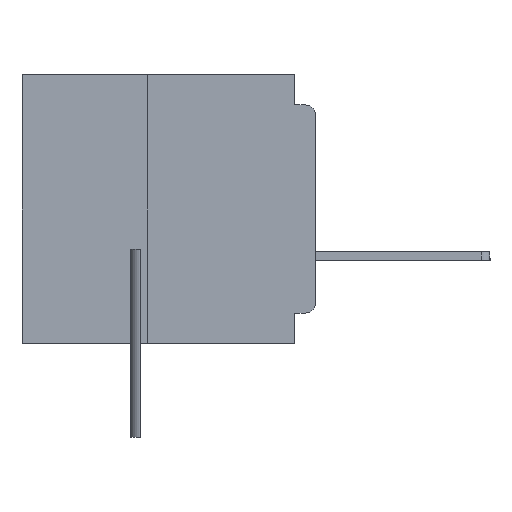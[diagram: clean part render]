
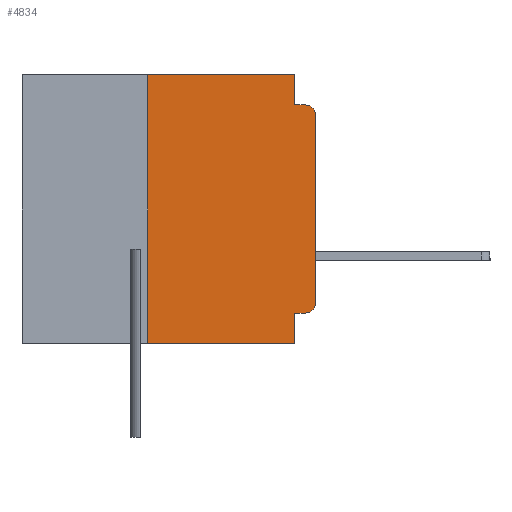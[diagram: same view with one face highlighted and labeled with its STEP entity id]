
A CAD part, left-side view. The second image highlights one B-rep face of the part: STEP entity #4834.
In plain terms, the highlighted planar face has unit normal (-1, 0, 0).
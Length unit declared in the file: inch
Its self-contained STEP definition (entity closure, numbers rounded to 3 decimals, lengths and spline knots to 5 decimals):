
#657 = VERTEX_POINT ( 'NONE', #24587 ) ;
#1069 = LINE ( 'NONE', #27262, #24691 ) ;
#2709 = VERTEX_POINT ( 'NONE', #43871 ) ;
#2829 = ORIENTED_EDGE ( 'NONE', *, *, #49684, .F. ) ;
#3603 = EDGE_LOOP ( 'NONE', ( #48235, #35257, #27024, #27379, #2829, #15830, #34248, #24601, #42728, #38411 ) ) ;
#3799 = CARTESIAN_POINT ( 'NONE',  ( 0., 0.015, -0.045 ) ) ;
#4523 = DIRECTION ( 'NONE',  ( 0., 1., 0. ) ) ;
#4640 = LINE ( 'NONE', #40777, #40723 ) ;
#4834 = ADVANCED_FACE ( 'NONE', ( #41984 ), #10911, .F. ) ;
#5202 = EDGE_CURVE ( 'NONE', #27704, #25353, #43397, .T. ) ;
#6354 = EDGE_CURVE ( 'NONE', #16294, #2709, #4640, .T. ) ;
#6828 = EDGE_CURVE ( 'NONE', #657, #21775, #26695, .T. ) ;
#6888 = CIRCLE ( 'NONE', #37696, 0.015 ) ;
#8313 = VERTEX_POINT ( 'NONE', #26538 ) ;
#8894 = LINE ( 'NONE', #42037, #44947 ) ;
#9525 = VECTOR ( 'NONE', #42294, 39.37008 ) ;
#9607 = LINE ( 'NONE', #11232, #58121 ) ;
#10692 = EDGE_CURVE ( 'NONE', #45711, #8313, #1069, .T. ) ;
#10911 = PLANE ( 'NONE',  #17857 ) ;
#11232 = CARTESIAN_POINT ( 'NONE',  ( 0., 0.437, 0. ) ) ;
#11774 = LINE ( 'NONE', #32186, #60242 ) ;
#12510 = LINE ( 'NONE', #23431, #9525 ) ;
#12685 = EDGE_CURVE ( 'NONE', #19572, #657, #8894, .T. ) ;
#12702 = VECTOR ( 'NONE', #43538, 39.37008 ) ;
#13257 = DIRECTION ( 'NONE',  ( 0., 0., -1. ) ) ;
#15384 = CARTESIAN_POINT ( 'NONE',  ( 0., 0., -0.045 ) ) ;
#15830 = ORIENTED_EDGE ( 'NONE', *, *, #6354, .F. ) ;
#16294 = VERTEX_POINT ( 'NONE', #21218 ) ;
#16322 = VERTEX_POINT ( 'NONE', #30908 ) ;
#17353 = DIRECTION ( 'NONE',  ( 0., 0., 1. ) ) ;
#17857 = AXIS2_PLACEMENT_3D ( 'NONE', #43813, #48544, #20377 ) ;
#18184 = DIRECTION ( 'NONE',  ( 0., -1., 0. ) ) ;
#18458 = DIRECTION ( 'NONE',  ( -1., 0., 0. ) ) ;
#19572 = VERTEX_POINT ( 'NONE', #23081 ) ;
#20377 = DIRECTION ( 'NONE',  ( 0., 0., -1. ) ) ;
#21218 = CARTESIAN_POINT ( 'NONE',  ( 0., 0.25, -0.4 ) ) ;
#21775 = VERTEX_POINT ( 'NONE', #3799 ) ;
#23081 = CARTESIAN_POINT ( 'NONE',  ( 0., 0.031, 0. ) ) ;
#23431 = CARTESIAN_POINT ( 'NONE',  ( 0., 0., 0. ) ) ;
#24587 = CARTESIAN_POINT ( 'NONE',  ( 0., 0.031, -0.045 ) ) ;
#24601 = ORIENTED_EDGE ( 'NONE', *, *, #10692, .F. ) ;
#24691 = VECTOR ( 'NONE', #13257, 39.37008 ) ;
#24970 = EDGE_CURVE ( 'NONE', #27704, #45711, #48728, .T. ) ;
#25353 = VERTEX_POINT ( 'NONE', #49555 ) ;
#26538 = CARTESIAN_POINT ( 'NONE',  ( 0., 0.031, -0.4 ) ) ;
#26695 = LINE ( 'NONE', #15384, #12702 ) ;
#27024 = ORIENTED_EDGE ( 'NONE', *, *, #6828, .F. ) ;
#27262 = CARTESIAN_POINT ( 'NONE',  ( 0., 0.031, -0.4 ) ) ;
#27379 = ORIENTED_EDGE ( 'NONE', *, *, #12685, .F. ) ;
#27704 = VERTEX_POINT ( 'NONE', #49880 ) ;
#28183 = DIRECTION ( 'NONE',  ( -1., 0., 0. ) ) ;
#30908 = CARTESIAN_POINT ( 'NONE',  ( 0., 0., -0.06 ) ) ;
#30952 = EDGE_CURVE ( 'NONE', #25353, #16322, #12510, .T. ) ;
#32186 = CARTESIAN_POINT ( 'NONE',  ( 0., 0.437, -0.4 ) ) ;
#32771 = CARTESIAN_POINT ( 'NONE',  ( 0., 0., -0.355 ) ) ;
#34248 = ORIENTED_EDGE ( 'NONE', *, *, #45353, .T. ) ;
#35257 = ORIENTED_EDGE ( 'NONE', *, *, #43048, .T. ) ;
#37332 = DIRECTION ( 'NONE',  ( 0., 0., -1. ) ) ;
#37695 = VECTOR ( 'NONE', #4523, 39.37008 ) ;
#37696 = AXIS2_PLACEMENT_3D ( 'NONE', #46581, #18458, #51332 ) ;
#38411 = ORIENTED_EDGE ( 'NONE', *, *, #5202, .T. ) ;
#40723 = VECTOR ( 'NONE', #17353, 39.37008 ) ;
#40777 = CARTESIAN_POINT ( 'NONE',  ( 0., 0.25, -0.4 ) ) ;
#41984 = FACE_OUTER_BOUND ( 'NONE', #3603, .T. ) ;
#42037 = CARTESIAN_POINT ( 'NONE',  ( 0., 0.031, 0. ) ) ;
#42294 = DIRECTION ( 'NONE',  ( 0., 0., 1. ) ) ;
#42728 = ORIENTED_EDGE ( 'NONE', *, *, #24970, .F. ) ;
#43048 = EDGE_CURVE ( 'NONE', #16322, #21775, #6888, .T. ) ;
#43397 = CIRCLE ( 'NONE', #48196, 0.015 ) ;
#43538 = DIRECTION ( 'NONE',  ( 0., -1., 0. ) ) ;
#43813 = CARTESIAN_POINT ( 'NONE',  ( 0., 0.437, 0. ) ) ;
#43871 = CARTESIAN_POINT ( 'NONE',  ( 0., 0.25, 0. ) ) ;
#44112 = DIRECTION ( 'NONE',  ( 0., -1., 0. ) ) ;
#44626 = CARTESIAN_POINT ( 'NONE',  ( 0., 0.031, -0.355 ) ) ;
#44947 = VECTOR ( 'NONE', #37332, 39.37008 ) ;
#45353 = EDGE_CURVE ( 'NONE', #16294, #8313, #11774, .T. ) ;
#45711 = VERTEX_POINT ( 'NONE', #44626 ) ;
#46581 = CARTESIAN_POINT ( 'NONE',  ( 0., 0.015, -0.06 ) ) ;
#48196 = AXIS2_PLACEMENT_3D ( 'NONE', #56277, #28183, #60963 ) ;
#48235 = ORIENTED_EDGE ( 'NONE', *, *, #30952, .T. ) ;
#48544 = DIRECTION ( 'NONE',  ( 1., 0., 0. ) ) ;
#48728 = LINE ( 'NONE', #32771, #37695 ) ;
#49555 = CARTESIAN_POINT ( 'NONE',  ( 0., 0., -0.34 ) ) ;
#49684 = EDGE_CURVE ( 'NONE', #2709, #19572, #9607, .T. ) ;
#49880 = CARTESIAN_POINT ( 'NONE',  ( 0., 0.015, -0.355 ) ) ;
#51332 = DIRECTION ( 'NONE',  ( 0., 0., -1. ) ) ;
#56277 = CARTESIAN_POINT ( 'NONE',  ( 0., 0.015, -0.34 ) ) ;
#58121 = VECTOR ( 'NONE', #44112, 39.37008 ) ;
#60242 = VECTOR ( 'NONE', #18184, 39.37008 ) ;
#60963 = DIRECTION ( 'NONE',  ( 0., 0., -1. ) ) ;
